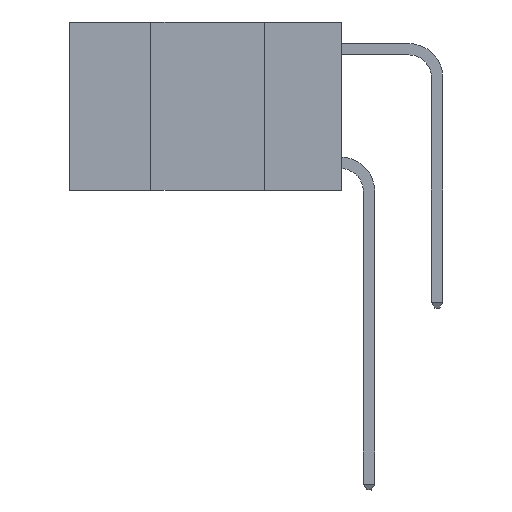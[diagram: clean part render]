
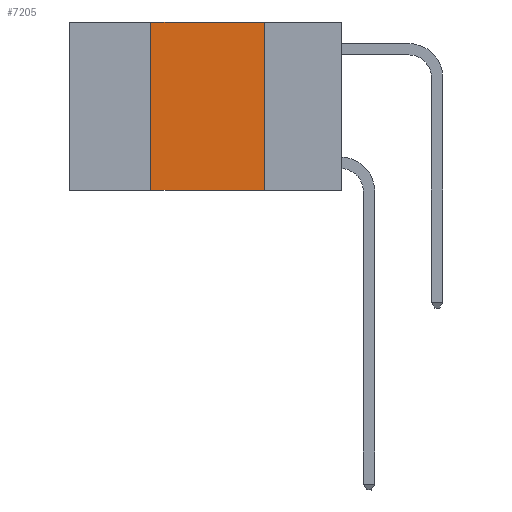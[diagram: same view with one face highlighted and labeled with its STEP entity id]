
A CAD part, left-side view. The second image highlights one B-rep face of the part: STEP entity #7205.
In plain terms, the highlighted planar face has unit normal (-1, 0, 0).
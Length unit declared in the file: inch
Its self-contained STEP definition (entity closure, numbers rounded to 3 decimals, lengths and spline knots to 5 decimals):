
#2184 = DIRECTION ( 'NONE',  ( 0., -1., 0. ) ) ;
#4558 = EDGE_CURVE ( 'NONE', #13761, #9231, #23594, .T. ) ;
#4736 = PLANE ( 'NONE',  #21277 ) ;
#5624 = EDGE_CURVE ( 'NONE', #15129, #26787, #29149, .T. ) ;
#6174 = DIRECTION ( 'NONE',  ( 0., -1., 0. ) ) ;
#7205 = ADVANCED_FACE ( 'NONE', ( #22633 ), #4736, .F. ) ;
#7388 = DIRECTION ( 'NONE',  ( 1., 0., 0. ) ) ;
#7833 = ORIENTED_EDGE ( 'NONE', *, *, #4558, .F. ) ;
#7952 = CARTESIAN_POINT ( 'NONE',  ( 0., 0.42, -0.37 ) ) ;
#9231 = VERTEX_POINT ( 'NONE', #28170 ) ;
#10691 = DIRECTION ( 'NONE',  ( 0., 0., 1. ) ) ;
#10819 = LINE ( 'NONE', #18776, #31365 ) ;
#12012 = LINE ( 'NONE', #15839, #18887 ) ;
#13761 = VERTEX_POINT ( 'NONE', #15798 ) ;
#14323 = VECTOR ( 'NONE', #2184, 39.37008 ) ;
#15129 = VERTEX_POINT ( 'NONE', #7952 ) ;
#15273 = CARTESIAN_POINT ( 'NONE',  ( 0., 0.6, 0. ) ) ;
#15798 = CARTESIAN_POINT ( 'NONE',  ( 0., 0.42, 0. ) ) ;
#15839 = CARTESIAN_POINT ( 'NONE',  ( 0., 0.42, 0. ) ) ;
#18776 = CARTESIAN_POINT ( 'NONE',  ( 0., 0.17, 0. ) ) ;
#18887 = VECTOR ( 'NONE', #10691, 39.37008 ) ;
#20325 = CARTESIAN_POINT ( 'NONE',  ( 0., 0.6, 0. ) ) ;
#20360 = CARTESIAN_POINT ( 'NONE',  ( 0., 0.17, -0.37 ) ) ;
#20401 = EDGE_LOOP ( 'NONE', ( #23883, #7833, #26581, #22236 ) ) ;
#21277 = AXIS2_PLACEMENT_3D ( 'NONE', #20325, #7388, #25513 ) ;
#21713 = CARTESIAN_POINT ( 'NONE',  ( 0., 0.6, -0.37 ) ) ;
#22236 = ORIENTED_EDGE ( 'NONE', *, *, #5624, .T. ) ;
#22633 = FACE_OUTER_BOUND ( 'NONE', #20401, .T. ) ;
#23594 = LINE ( 'NONE', #15273, #14323 ) ;
#23861 = DIRECTION ( 'NONE',  ( 0., 0., -1. ) ) ;
#23883 = ORIENTED_EDGE ( 'NONE', *, *, #26896, .F. ) ;
#23963 = VECTOR ( 'NONE', #6174, 39.37008 ) ;
#25513 = DIRECTION ( 'NONE',  ( 0., 0., -1. ) ) ;
#26581 = ORIENTED_EDGE ( 'NONE', *, *, #27516, .F. ) ;
#26787 = VERTEX_POINT ( 'NONE', #20360 ) ;
#26896 = EDGE_CURVE ( 'NONE', #9231, #26787, #10819, .T. ) ;
#27516 = EDGE_CURVE ( 'NONE', #15129, #13761, #12012, .T. ) ;
#28170 = CARTESIAN_POINT ( 'NONE',  ( 0., 0.17, 0. ) ) ;
#29149 = LINE ( 'NONE', #21713, #23963 ) ;
#31365 = VECTOR ( 'NONE', #23861, 39.37008 ) ;
